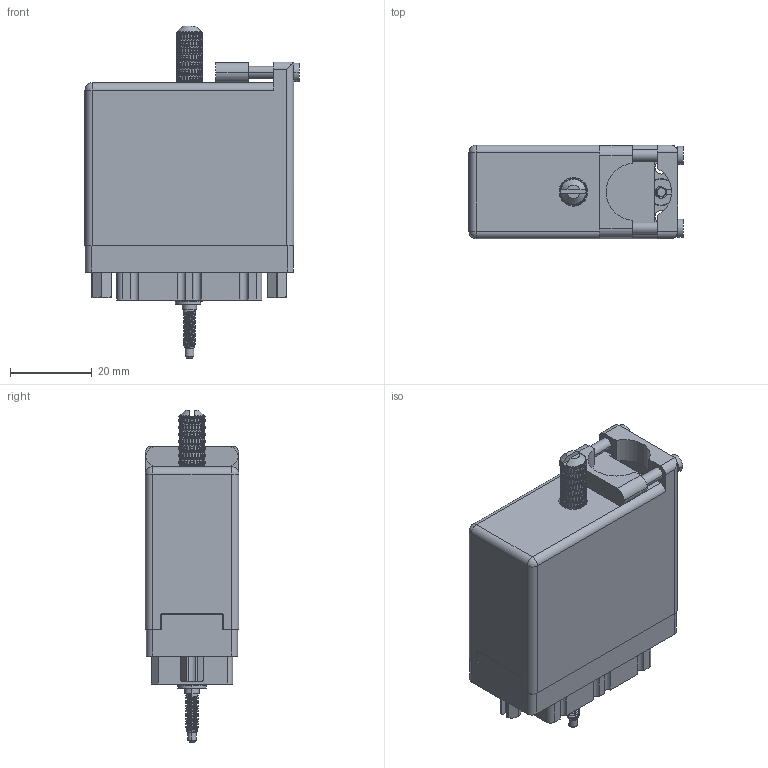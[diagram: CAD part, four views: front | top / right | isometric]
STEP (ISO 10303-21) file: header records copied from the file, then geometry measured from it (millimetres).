
FILE_DESCRIPTION (( 'STEP AP203' ), '1' );
FILE_NAME ('519-036-000-461.STEP', '2020-09-09T20:07:23', ( '' ), ( '' ), 'SwSTEP 2.0', 'SolidWorks 2020', '' );
FILE_SCHEMA (( 'CONFIG_CONTROL_DESIGN' ));
Length unit declared in the file: inch
Products named in the file (11): 516-252-021-102_038; 516-250-038-111; 519 Receptacle Insulator_036; 519-036-000-461; 516-230-001_Metal - 038 Top Entry; 516-253-138-107; 516-221-038-102_039; 516-251-035-100; 516-253-035-100; Actuating Screw Assy 038-056; 516-221-038-102_038
Assembly tree (12 placements, depth 3):
  519-036-000-461
    519 Receptacle Insulator_036
    Actuating Screw Assy 038-056
      516-251-035-100
      516-253-035-100  x2
      516-253-138-107
      516-250-038-111
    516-252-021-102_038  x2
    516-221-038-102_038
    516-221-038-102_039
    516-230-001_Metal - 038 Top Entry
Bounding box: 52.27 x 22.83 x 81.03 mm (x, y, z)
Volume: 22632.7 mm3; surface area: 31154.2 mm2
Topology: 11 solids, 11 shells, 2477 faces, 6113 edges, 3672 vertices
Faces by surface type: bspline 1034, plane 767, cylinder 622, cone 52, sphere 2
Entity records: 106049 total; most frequent: CARTESIAN_POINT 58820, ORIENTED_EDGE 12010, DIRECTION 6976, EDGE_CURVE 6005, VERTEX_POINT 3604, EDGE_LOOP 2563, FACE_OUTER_BOUND 2440, ADVANCED_FACE 2440
